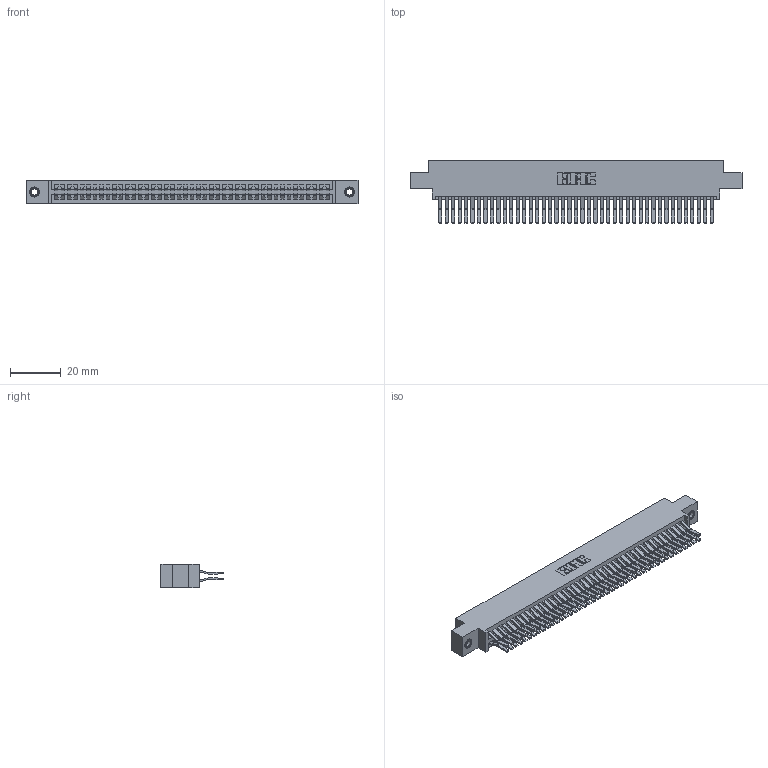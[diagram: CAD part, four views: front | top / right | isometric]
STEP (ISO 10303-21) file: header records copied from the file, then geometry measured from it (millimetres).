
FILE_DESCRIPTION (( 'STEP AP203' ), '1' );
FILE_NAME ('395-086-560-807.STEP', '2019-10-25T13:05:00', ( '' ), ( '' ), 'SwSTEP 2.0', 'SolidWorks 2016', '' );
FILE_SCHEMA (( 'CONFIG_CONTROL_DESIGN' ));
Length unit declared in the file: inch
Products named in the file (4): 395-086-560-807; 345 Part_0.170 Offset - 0.156 Dia-TI; 345-292-001_560 Tail; 345-250-001_345-250-005-103
Assembly tree (89 placements, depth 2):
  395-086-560-807
    345 Part_0.170 Offset - 0.156 Dia-TI
    345-292-001_560 Tail  x86
    345-250-001_345-250-005-103  x2
Bounding box: 130.43 x 24.45 x 9.4 mm (x, y, z)
Volume: 13116.1 mm3; surface area: 21028.3 mm2
Topology: 89 solids, 89 shells, 4662 faces, 13819 edges, 9090 vertices
Faces by surface type: plane 2954, cylinder 1692, cone 12, torus 4
Entity records: 35010 total; most frequent: CARTESIAN_POINT 5851, ORIENTED_EDGE 5778, DIRECTION 5187, EDGE_CURVE 2889, VECTOR 2561, LINE 2561, VERTEX_POINT 1920, AXIS2_PLACEMENT_3D 1313
